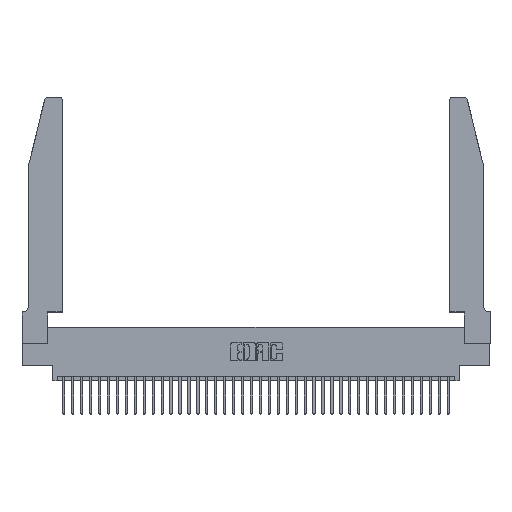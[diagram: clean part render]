
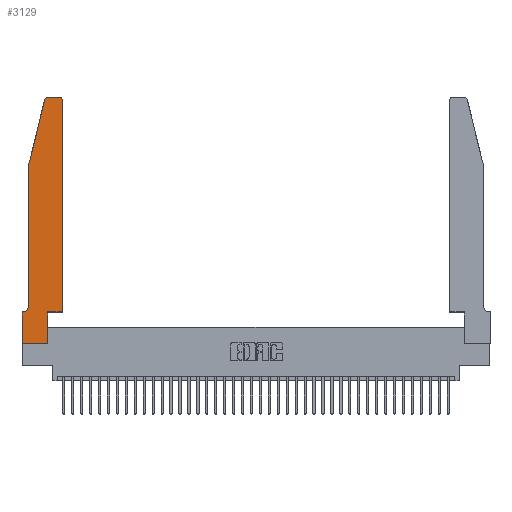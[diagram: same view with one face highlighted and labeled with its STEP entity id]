
A CAD part, top view. The second image highlights one B-rep face of the part: STEP entity #3129.
In plain terms, the highlighted planar face has unit normal (0, 0, 1).
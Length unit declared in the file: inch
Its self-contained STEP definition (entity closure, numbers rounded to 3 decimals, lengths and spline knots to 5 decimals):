
#37 = DIRECTION ( 'NONE',  ( 1., 0., 0. ) ) ;
#800 = CARTESIAN_POINT ( 'NONE',  ( 0.2605, 2.75, 0.37 ) ) ;
#1741 = VERTEX_POINT ( 'NONE', #30318 ) ;
#3129 = ADVANCED_FACE ( 'NONE', ( #13532 ), #13165, .T. ) ;
#3221 = ORIENTED_EDGE ( 'NONE', *, *, #7628, .T. ) ;
#3613 = EDGE_CURVE ( 'NONE', #26190, #7489, #29637, .T. ) ;
#4331 = CARTESIAN_POINT ( 'NONE',  ( 0.284, 2.75, 0.37 ) ) ;
#5078 = EDGE_CURVE ( 'NONE', #7489, #26276, #25742, .T. ) ;
#5571 = ORIENTED_EDGE ( 'NONE', *, *, #25267, .T. ) ;
#5920 = DIRECTION ( 'NONE',  ( 0., 0., 1. ) ) ;
#6019 = VECTOR ( 'NONE', #14018, 39.37008 ) ;
#6127 = AXIS2_PLACEMENT_3D ( 'NONE', #36310, #18220, #37 ) ;
#6646 = CARTESIAN_POINT ( 'NONE',  ( 0.0755, 2., 0.37 ) ) ;
#6729 = DIRECTION ( 'NONE',  ( -1., 0., 0. ) ) ;
#6842 = VERTEX_POINT ( 'NONE', #24545 ) ;
#6883 = CARTESIAN_POINT ( 'NONE',  ( 0.4505, 0.35, 0.37 ) ) ;
#7267 = CARTESIAN_POINT ( 'NONE',  ( 0., 0.35, 0.37 ) ) ;
#7489 = VERTEX_POINT ( 'NONE', #33563 ) ;
#7566 = VERTEX_POINT ( 'NONE', #24891 ) ;
#7628 = EDGE_CURVE ( 'NONE', #25266, #7566, #24290, .T. ) ;
#7712 = VERTEX_POINT ( 'NONE', #7267 ) ;
#8068 = VECTOR ( 'NONE', #34072, 39.37008 ) ;
#8764 = EDGE_CURVE ( 'NONE', #7712, #27112, #23227, .T. ) ;
#9424 = ORIENTED_EDGE ( 'NONE', *, *, #11585, .T. ) ;
#9542 = VECTOR ( 'NONE', #21850, 39.37008 ) ;
#9982 = DIRECTION ( 'NONE',  ( 1., 0., 0. ) ) ;
#10643 = VERTEX_POINT ( 'NONE', #32171 ) ;
#11139 = VECTOR ( 'NONE', #6729, 39.37008 ) ;
#11585 = EDGE_CURVE ( 'NONE', #10643, #25266, #29674, .T. ) ;
#11718 = VECTOR ( 'NONE', #15629, 39.37008 ) ;
#11812 = ORIENTED_EDGE ( 'NONE', *, *, #21114, .T. ) ;
#12201 = DIRECTION ( 'NONE',  ( -0.239, -0.971, 0. ) ) ;
#13026 = VECTOR ( 'NONE', #17676, 39.37008 ) ;
#13165 = PLANE ( 'NONE',  #36822 ) ;
#13234 = ORIENTED_EDGE ( 'NONE', *, *, #26406, .T. ) ;
#13311 = EDGE_LOOP ( 'NONE', ( #13234, #29374, #17033, #34990, #11812, #5571, #37812, #14675, #16579, #9424, #3221, #37356 ) ) ;
#13532 = FACE_OUTER_BOUND ( 'NONE', #13311, .T. ) ;
#14018 = DIRECTION ( 'NONE',  ( 0., -1., 0. ) ) ;
#14638 = CARTESIAN_POINT ( 'NONE',  ( 0.2865, 0.35, 0.37 ) ) ;
#14675 = ORIENTED_EDGE ( 'NONE', *, *, #21989, .T. ) ;
#14782 = CARTESIAN_POINT ( 'NONE',  ( 0.25487, 2.72718, 0.37 ) ) ;
#15190 = CARTESIAN_POINT ( 'NONE',  ( 0., 0., 0.37 ) ) ;
#15497 = CARTESIAN_POINT ( 'NONE',  ( 0.4505, 0.35, 0.37 ) ) ;
#15629 = DIRECTION ( 'NONE',  ( -1., 0., 0. ) ) ;
#15965 = CARTESIAN_POINT ( 'NONE',  ( 0.4505, 0.35, 0.37 ) ) ;
#16182 = EDGE_CURVE ( 'NONE', #7566, #36266, #37345, .T. ) ;
#16217 = CARTESIAN_POINT ( 'NONE',  ( 0., 0.35, 0.37 ) ) ;
#16579 = ORIENTED_EDGE ( 'NONE', *, *, #35155, .T. ) ;
#17033 = ORIENTED_EDGE ( 'NONE', *, *, #3613, .T. ) ;
#17676 = DIRECTION ( 'NONE',  ( 0., 1., 0. ) ) ;
#17769 = CARTESIAN_POINT ( 'NONE',  ( 0.0055, 0.42, 0.37 ) ) ;
#18220 = DIRECTION ( 'NONE',  ( 0., 0., 1. ) ) ;
#19079 = VECTOR ( 'NONE', #27424, 39.37008 ) ;
#19241 = DIRECTION ( 'NONE',  ( 1., 0., 0. ) ) ;
#20175 = LINE ( 'NONE', #800, #11139 ) ;
#20488 = EDGE_CURVE ( 'NONE', #20839, #26190, #28661, .T. ) ;
#20812 = DIRECTION ( 'NONE',  ( -1., 0., 0. ) ) ;
#20839 = VERTEX_POINT ( 'NONE', #4331 ) ;
#21114 = EDGE_CURVE ( 'NONE', #26276, #1741, #31903, .T. ) ;
#21138 = CARTESIAN_POINT ( 'NONE',  ( 0.0755, 0.42, 0.37 ) ) ;
#21606 = VECTOR ( 'NONE', #9982, 39.37008 ) ;
#21850 = DIRECTION ( 'NONE',  ( 0., -1., 0. ) ) ;
#21989 = EDGE_CURVE ( 'NONE', #27112, #6842, #27207, .T. ) ;
#23227 = LINE ( 'NONE', #35142, #6019 ) ;
#24214 = CARTESIAN_POINT ( 'NONE',  ( 0.284, 2.72, 0.37 ) ) ;
#24290 = LINE ( 'NONE', #15965, #8068 ) ;
#24545 = CARTESIAN_POINT ( 'NONE',  ( 0.2865, 0., 0.37 ) ) ;
#24891 = CARTESIAN_POINT ( 'NONE',  ( 0.4505, 2.72, 0.37 ) ) ;
#25266 = VERTEX_POINT ( 'NONE', #15497 ) ;
#25267 = EDGE_CURVE ( 'NONE', #1741, #7712, #35836, .T. ) ;
#25742 = LINE ( 'NONE', #6646, #9542 ) ;
#26190 = VERTEX_POINT ( 'NONE', #14782 ) ;
#26276 = VERTEX_POINT ( 'NONE', #21138 ) ;
#26406 = EDGE_CURVE ( 'NONE', #36266, #20839, #20175, .T. ) ;
#26537 = CARTESIAN_POINT ( 'NONE',  ( 0.4205, 2.75, 0.37 ) ) ;
#26726 = AXIS2_PLACEMENT_3D ( 'NONE', #17769, #38859, #20812 ) ;
#27112 = VERTEX_POINT ( 'NONE', #31161 ) ;
#27207 = LINE ( 'NONE', #15190, #19079 ) ;
#27255 = DIRECTION ( 'NONE',  ( 1., 0., 0. ) ) ;
#27424 = DIRECTION ( 'NONE',  ( 1., 0., 0. ) ) ;
#28661 = CIRCLE ( 'NONE', #34222, 0.03 ) ;
#29374 = ORIENTED_EDGE ( 'NONE', *, *, #20488, .T. ) ;
#29637 = LINE ( 'NONE', #36398, #37585 ) ;
#29674 = LINE ( 'NONE', #6883, #21606 ) ;
#30318 = CARTESIAN_POINT ( 'NONE',  ( 0.0055, 0.35, 0.37 ) ) ;
#30748 = CARTESIAN_POINT ( 'NONE',  ( 0.0755, 0.35, 0.37 ) ) ;
#31161 = CARTESIAN_POINT ( 'NONE',  ( 0., 0., 0.37 ) ) ;
#31903 = CIRCLE ( 'NONE', #26726, 0.07 ) ;
#32171 = CARTESIAN_POINT ( 'NONE',  ( 0.2865, 0.35, 0.37 ) ) ;
#33563 = CARTESIAN_POINT ( 'NONE',  ( 0.0755, 2., 0.37 ) ) ;
#34072 = DIRECTION ( 'NONE',  ( 0., 1., 0. ) ) ;
#34222 = AXIS2_PLACEMENT_3D ( 'NONE', #24214, #5920, #27255 ) ;
#34990 = ORIENTED_EDGE ( 'NONE', *, *, #5078, .T. ) ;
#35142 = CARTESIAN_POINT ( 'NONE',  ( 0., 0., 0.37 ) ) ;
#35155 = EDGE_CURVE ( 'NONE', #6842, #10643, #37121, .T. ) ;
#35836 = LINE ( 'NONE', #30748, #11718 ) ;
#36266 = VERTEX_POINT ( 'NONE', #26537 ) ;
#36310 = CARTESIAN_POINT ( 'NONE',  ( 0.4205, 2.72, 0.37 ) ) ;
#36398 = CARTESIAN_POINT ( 'NONE',  ( 0.0755, 2., 0.37 ) ) ;
#36822 = AXIS2_PLACEMENT_3D ( 'NONE', #16217, #37324, #19241 ) ;
#37121 = LINE ( 'NONE', #14638, #13026 ) ;
#37324 = DIRECTION ( 'NONE',  ( 0., 0., 1. ) ) ;
#37345 = CIRCLE ( 'NONE', #6127, 0.03 ) ;
#37356 = ORIENTED_EDGE ( 'NONE', *, *, #16182, .T. ) ;
#37585 = VECTOR ( 'NONE', #12201, 39.37008 ) ;
#37812 = ORIENTED_EDGE ( 'NONE', *, *, #8764, .T. ) ;
#38859 = DIRECTION ( 'NONE',  ( 0., 0., -1. ) ) ;
